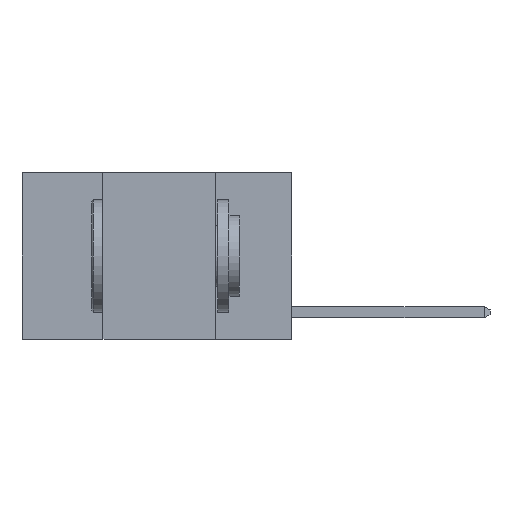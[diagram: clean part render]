
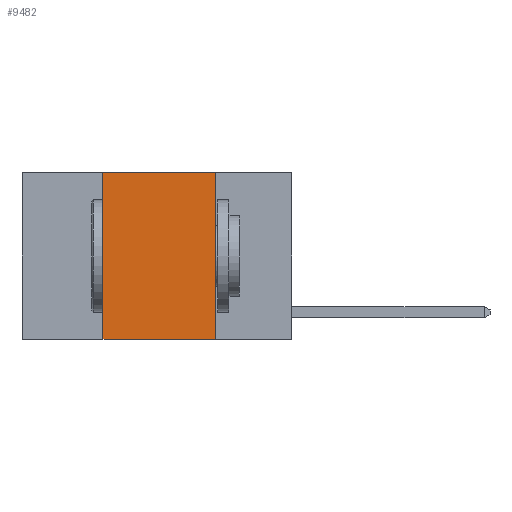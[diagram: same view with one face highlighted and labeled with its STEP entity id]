
A CAD part, left-side view. The second image highlights one B-rep face of the part: STEP entity #9482.
In plain terms, the highlighted planar face has unit normal (-1, 0, 0).
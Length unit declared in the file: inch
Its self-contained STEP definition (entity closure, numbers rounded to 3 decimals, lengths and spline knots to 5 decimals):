
#137 = EDGE_CURVE ( 'NONE', #1804, #9082, #1188, .T. ) ;
#210 = VECTOR ( 'NONE', #6029, 39.37008 ) ;
#523 = VERTEX_POINT ( 'NONE', #9714 ) ;
#836 = DIRECTION ( 'NONE',  ( 0., -1., 0. ) ) ;
#960 = CARTESIAN_POINT ( 'NONE',  ( 0., 0.6, -0.37 ) ) ;
#1188 = LINE ( 'NONE', #5999, #7855 ) ;
#1245 = CARTESIAN_POINT ( 'NONE',  ( 0., 0.42, 0. ) ) ;
#1427 = VECTOR ( 'NONE', #10685, 39.37008 ) ;
#1538 = CARTESIAN_POINT ( 'NONE',  ( 0., 0.6, 0. ) ) ;
#1691 = DIRECTION ( 'NONE',  ( 0., 0., -1. ) ) ;
#1724 = LINE ( 'NONE', #1973, #1427 ) ;
#1804 = VERTEX_POINT ( 'NONE', #2663 ) ;
#1924 = ORIENTED_EDGE ( 'NONE', *, *, #2776, .F. ) ;
#1973 = CARTESIAN_POINT ( 'NONE',  ( 0., 0.17, 0. ) ) ;
#1989 = EDGE_LOOP ( 'NONE', ( #1924, #3673, #10127, #9657 ) ) ;
#2178 = VECTOR ( 'NONE', #836, 39.37008 ) ;
#2638 = LINE ( 'NONE', #1538, #210 ) ;
#2663 = CARTESIAN_POINT ( 'NONE',  ( 0., 0.42, -0.37 ) ) ;
#2776 = EDGE_CURVE ( 'NONE', #523, #9084, #1724, .T. ) ;
#2937 = EDGE_CURVE ( 'NONE', #1804, #9084, #8625, .T. ) ;
#3673 = ORIENTED_EDGE ( 'NONE', *, *, #6704, .F. ) ;
#5999 = CARTESIAN_POINT ( 'NONE',  ( 0., 0.42, 0. ) ) ;
#6029 = DIRECTION ( 'NONE',  ( 0., -1., 0. ) ) ;
#6121 = CARTESIAN_POINT ( 'NONE',  ( 0., 0.6, 0. ) ) ;
#6704 = EDGE_CURVE ( 'NONE', #9082, #523, #2638, .T. ) ;
#6780 = FACE_OUTER_BOUND ( 'NONE', #1989, .T. ) ;
#6943 = DIRECTION ( 'NONE',  ( 1., 0., 0. ) ) ;
#7364 = CARTESIAN_POINT ( 'NONE',  ( 0., 0.17, -0.37 ) ) ;
#7855 = VECTOR ( 'NONE', #9380, 39.37008 ) ;
#7890 = AXIS2_PLACEMENT_3D ( 'NONE', #6121, #6943, #1691 ) ;
#8625 = LINE ( 'NONE', #960, #2178 ) ;
#9082 = VERTEX_POINT ( 'NONE', #1245 ) ;
#9084 = VERTEX_POINT ( 'NONE', #7364 ) ;
#9380 = DIRECTION ( 'NONE',  ( 0., 0., 1. ) ) ;
#9482 = ADVANCED_FACE ( 'NONE', ( #6780 ), #10748, .F. ) ;
#9657 = ORIENTED_EDGE ( 'NONE', *, *, #2937, .T. ) ;
#9714 = CARTESIAN_POINT ( 'NONE',  ( 0., 0.17, 0. ) ) ;
#10127 = ORIENTED_EDGE ( 'NONE', *, *, #137, .F. ) ;
#10685 = DIRECTION ( 'NONE',  ( 0., 0., -1. ) ) ;
#10748 = PLANE ( 'NONE',  #7890 ) ;
